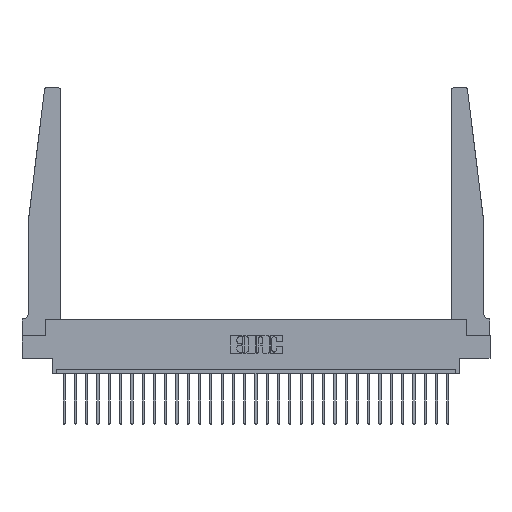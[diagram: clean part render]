
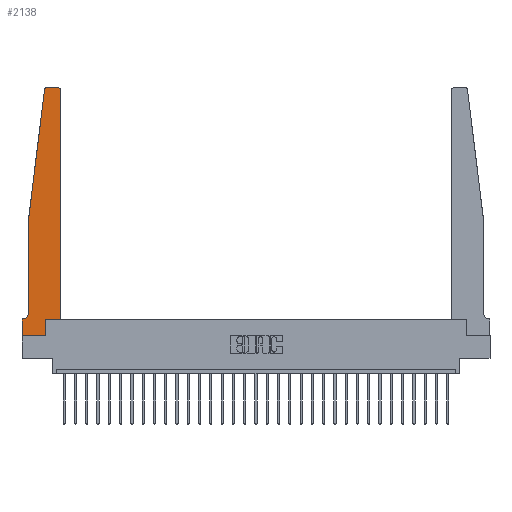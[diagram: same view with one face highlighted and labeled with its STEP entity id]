
A CAD part, top view. The second image highlights one B-rep face of the part: STEP entity #2138.
In plain terms, the highlighted planar face has unit normal (0, 0, 1).
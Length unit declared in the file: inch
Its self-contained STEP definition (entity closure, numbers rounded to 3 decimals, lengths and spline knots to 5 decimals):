
#193 = ORIENTED_EDGE ( 'NONE', *, *, #11389, .T. ) ;
#685 = EDGE_CURVE ( 'NONE', #5642, #18323, #6851, .T. ) ;
#890 = ORIENTED_EDGE ( 'NONE', *, *, #8434, .T. ) ;
#1243 = ORIENTED_EDGE ( 'NONE', *, *, #7207, .T. ) ;
#1374 = AXIS2_PLACEMENT_3D ( 'NONE', #19983, #15046, #6669 ) ;
#1428 = VERTEX_POINT ( 'NONE', #15968 ) ;
#1823 = DIRECTION ( 'NONE',  ( 1., 0., 0. ) ) ;
#2003 = LINE ( 'NONE', #19009, #12233 ) ;
#2052 = DIRECTION ( 'NONE',  ( 1., 0., 0. ) ) ;
#2080 = ORIENTED_EDGE ( 'NONE', *, *, #15644, .T. ) ;
#2138 = ADVANCED_FACE ( 'NONE', ( #21747 ), #19732, .T. ) ;
#2161 = VECTOR ( 'NONE', #14916, 39.37008 ) ;
#2308 = VECTOR ( 'NONE', #5431, 39.37008 ) ;
#2584 = ORIENTED_EDGE ( 'NONE', *, *, #5209, .T. ) ;
#2703 = CARTESIAN_POINT ( 'NONE',  ( 0., 0.1875, 0.37 ) ) ;
#2726 = ORIENTED_EDGE ( 'NONE', *, *, #3780, .T. ) ;
#2941 = EDGE_CURVE ( 'NONE', #15798, #5642, #20622, .T. ) ;
#3149 = CARTESIAN_POINT ( 'NONE',  ( 0.425, 2.72, 0.37 ) ) ;
#3648 = VERTEX_POINT ( 'NONE', #6949 ) ;
#3698 = AXIS2_PLACEMENT_3D ( 'NONE', #3956, #23546, #1823 ) ;
#3702 = VERTEX_POINT ( 'NONE', #9243 ) ;
#3780 = EDGE_CURVE ( 'NONE', #5128, #19878, #23588, .T. ) ;
#3956 = CARTESIAN_POINT ( 'NONE',  ( 0.395, 2.72, 0.37 ) ) ;
#4115 = LINE ( 'NONE', #12796, #2161 ) ;
#4497 = CARTESIAN_POINT ( 'NONE',  ( 0.425, 0.18, 0.37 ) ) ;
#5073 = VECTOR ( 'NONE', #18038, 39.37008 ) ;
#5128 = VERTEX_POINT ( 'NONE', #5595 ) ;
#5209 = EDGE_CURVE ( 'NONE', #3702, #19186, #24794, .T. ) ;
#5217 = ORIENTED_EDGE ( 'NONE', *, *, #26299, .T. ) ;
#5431 = DIRECTION ( 'NONE',  ( 0., 1., 0. ) ) ;
#5595 = CARTESIAN_POINT ( 'NONE',  ( 0.065, 0.2375, 0.37 ) ) ;
#5642 = VERTEX_POINT ( 'NONE', #25707 ) ;
#6272 = CARTESIAN_POINT ( 'NONE',  ( 0.2605, 0., 0.37 ) ) ;
#6591 = CARTESIAN_POINT ( 'NONE',  ( 0.395, 2.75, 0.37 ) ) ;
#6669 = DIRECTION ( 'NONE',  ( -1., 0., 0. ) ) ;
#6690 = DIRECTION ( 'NONE',  ( 1., 0., 0. ) ) ;
#6851 = LINE ( 'NONE', #26290, #27864 ) ;
#6949 = CARTESIAN_POINT ( 'NONE',  ( 0.065, 1.25, 0.37 ) ) ;
#7207 = EDGE_CURVE ( 'NONE', #19240, #3702, #4115, .T. ) ;
#7277 = VECTOR ( 'NONE', #20489, 39.37008 ) ;
#7917 = CARTESIAN_POINT ( 'NONE',  ( 0.065, 1.25, 0.37 ) ) ;
#8294 = VERTEX_POINT ( 'NONE', #3149 ) ;
#8434 = EDGE_CURVE ( 'NONE', #1428, #15798, #2003, .T. ) ;
#9243 = CARTESIAN_POINT ( 'NONE',  ( 0.27653, 2.75, 0.37 ) ) ;
#9526 = AXIS2_PLACEMENT_3D ( 'NONE', #15623, #21890, #6690 ) ;
#10615 = VECTOR ( 'NONE', #13135, 39.37008 ) ;
#10964 = CIRCLE ( 'NONE', #3698, 0.03 ) ;
#10981 = VECTOR ( 'NONE', #15420, 39.37008 ) ;
#10995 = VECTOR ( 'NONE', #23099, 39.37008 ) ;
#11389 = EDGE_CURVE ( 'NONE', #26775, #1428, #13000, .T. ) ;
#11853 = LINE ( 'NONE', #14127, #7277 ) ;
#11991 = CARTESIAN_POINT ( 'NONE',  ( 0.2605, 0.18, 0.37 ) ) ;
#12233 = VECTOR ( 'NONE', #27956, 39.37008 ) ;
#12796 = CARTESIAN_POINT ( 'NONE',  ( 0.25, 2.75, 0.37 ) ) ;
#13000 = LINE ( 'NONE', #21648, #10615 ) ;
#13135 = DIRECTION ( 'NONE',  ( 0., -1., 0. ) ) ;
#13907 = CARTESIAN_POINT ( 'NONE',  ( 0.015, 0.1875, 0.37 ) ) ;
#13958 = ORIENTED_EDGE ( 'NONE', *, *, #15951, .T. ) ;
#14127 = CARTESIAN_POINT ( 'NONE',  ( 0.065, 1.25, 0.37 ) ) ;
#14639 = CARTESIAN_POINT ( 'NONE',  ( 0.425, 0.18, 0.37 ) ) ;
#14849 = LINE ( 'NONE', #7917, #10995 ) ;
#14916 = DIRECTION ( 'NONE',  ( -1., 0., 0. ) ) ;
#15046 = DIRECTION ( 'NONE',  ( 0., 0., -1. ) ) ;
#15124 = CARTESIAN_POINT ( 'NONE',  ( 0.065, 0.1875, 0.37 ) ) ;
#15420 = DIRECTION ( 'NONE',  ( 0., 1., 0. ) ) ;
#15623 = CARTESIAN_POINT ( 'NONE',  ( 0., 0.1875, 0.37 ) ) ;
#15644 = EDGE_CURVE ( 'NONE', #19186, #3648, #11853, .T. ) ;
#15798 = VERTEX_POINT ( 'NONE', #6272 ) ;
#15951 = EDGE_CURVE ( 'NONE', #8294, #19240, #10964, .T. ) ;
#15968 = CARTESIAN_POINT ( 'NONE',  ( 0., 0., 0.37 ) ) ;
#17391 = ORIENTED_EDGE ( 'NONE', *, *, #685, .T. ) ;
#18038 = DIRECTION ( 'NONE',  ( -1., 0., 0. ) ) ;
#18323 = VERTEX_POINT ( 'NONE', #14639 ) ;
#19009 = CARTESIAN_POINT ( 'NONE',  ( 0., 0., 0.37 ) ) ;
#19186 = VERTEX_POINT ( 'NONE', #27180 ) ;
#19191 = DIRECTION ( 'NONE',  ( 0., 0., 1. ) ) ;
#19240 = VERTEX_POINT ( 'NONE', #6591 ) ;
#19732 = PLANE ( 'NONE',  #9526 ) ;
#19751 = DIRECTION ( 'NONE',  ( 1., 0., 0. ) ) ;
#19878 = VERTEX_POINT ( 'NONE', #13907 ) ;
#19983 = CARTESIAN_POINT ( 'NONE',  ( 0.015, 0.2375, 0.37 ) ) ;
#20263 = ORIENTED_EDGE ( 'NONE', *, *, #26192, .T. ) ;
#20489 = DIRECTION ( 'NONE',  ( -0.122, -0.992, 0. ) ) ;
#20622 = LINE ( 'NONE', #11991, #2308 ) ;
#21531 = ORIENTED_EDGE ( 'NONE', *, *, #24186, .T. ) ;
#21648 = CARTESIAN_POINT ( 'NONE',  ( 0., 0., 0.37 ) ) ;
#21747 = FACE_OUTER_BOUND ( 'NONE', #26953, .T. ) ;
#21890 = DIRECTION ( 'NONE',  ( 0., 0., 1. ) ) ;
#22985 = AXIS2_PLACEMENT_3D ( 'NONE', #25475, #19191, #2052 ) ;
#23099 = DIRECTION ( 'NONE',  ( 0., -1., 0. ) ) ;
#23546 = DIRECTION ( 'NONE',  ( 0., 0., 1. ) ) ;
#23588 = CIRCLE ( 'NONE', #1374, 0.05 ) ;
#23647 = LINE ( 'NONE', #15124, #5073 ) ;
#24186 = EDGE_CURVE ( 'NONE', #18323, #8294, #26206, .T. ) ;
#24794 = CIRCLE ( 'NONE', #22985, 0.03 ) ;
#25475 = CARTESIAN_POINT ( 'NONE',  ( 0.27653, 2.72, 0.37 ) ) ;
#25707 = CARTESIAN_POINT ( 'NONE',  ( 0.2605, 0.18, 0.37 ) ) ;
#25802 = ORIENTED_EDGE ( 'NONE', *, *, #2941, .T. ) ;
#26192 = EDGE_CURVE ( 'NONE', #3648, #5128, #14849, .T. ) ;
#26206 = LINE ( 'NONE', #4497, #10981 ) ;
#26290 = CARTESIAN_POINT ( 'NONE',  ( 0.425, 0.18, 0.37 ) ) ;
#26299 = EDGE_CURVE ( 'NONE', #19878, #26775, #23647, .T. ) ;
#26775 = VERTEX_POINT ( 'NONE', #2703 ) ;
#26953 = EDGE_LOOP ( 'NONE', ( #1243, #2584, #2080, #20263, #2726, #5217, #193, #890, #25802, #17391, #21531, #13958 ) ) ;
#27180 = CARTESIAN_POINT ( 'NONE',  ( 0.24675, 2.72367, 0.37 ) ) ;
#27864 = VECTOR ( 'NONE', #19751, 39.37008 ) ;
#27956 = DIRECTION ( 'NONE',  ( 1., 0., 0. ) ) ;
